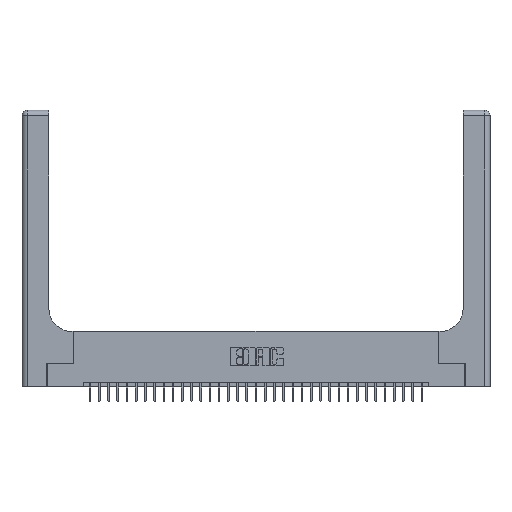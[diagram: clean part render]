
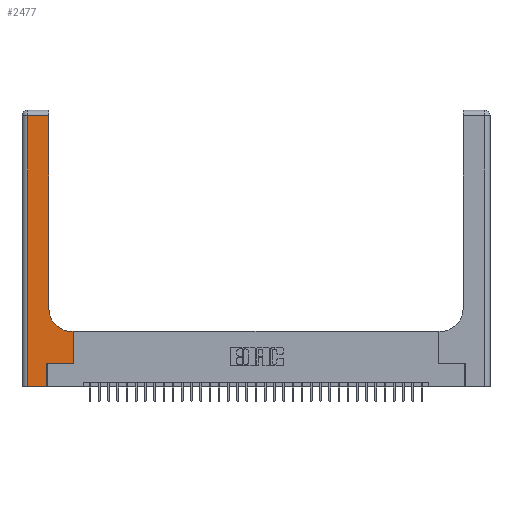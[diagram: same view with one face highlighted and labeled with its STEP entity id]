
A CAD part, top view. The second image highlights one B-rep face of the part: STEP entity #2477.
In plain terms, the highlighted planar face has unit normal (0, 0, 1).
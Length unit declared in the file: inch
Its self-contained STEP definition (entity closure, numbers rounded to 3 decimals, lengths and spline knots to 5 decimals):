
#260 = VERTEX_POINT ( 'NONE', #7170 ) ;
#374 = FACE_OUTER_BOUND ( 'NONE', #23663, .T. ) ;
#386 = VECTOR ( 'NONE', #18482, 39.37008 ) ;
#395 = ORIENTED_EDGE ( 'NONE', *, *, #7590, .T. ) ;
#452 = EDGE_CURVE ( 'NONE', #22883, #260, #27419, .T. ) ;
#1075 = DIRECTION ( 'NONE',  ( -1., 0., 0. ) ) ;
#1401 = CARTESIAN_POINT ( 'NONE',  ( 0.2915, 0.85, 0.37 ) ) ;
#1959 = EDGE_CURVE ( 'NONE', #24616, #23981, #8615, .T. ) ;
#2477 = ADVANCED_FACE ( 'NONE', ( #374 ), #9264, .F. ) ;
#3074 = EDGE_CURVE ( 'NONE', #260, #7965, #32493, .T. ) ;
#3697 = LINE ( 'NONE', #11061, #11027 ) ;
#3730 = DIRECTION ( 'NONE',  ( 0., 1., 0. ) ) ;
#3807 = CARTESIAN_POINT ( 'NONE',  ( 0.269, 0., 0.37 ) ) ;
#4621 = VECTOR ( 'NONE', #12087, 39.37008 ) ;
#4744 = EDGE_CURVE ( 'NONE', #23981, #9848, #3697, .T. ) ;
#5275 = CARTESIAN_POINT ( 'NONE',  ( 0.5585, 0.6, 0.37 ) ) ;
#6209 = CARTESIAN_POINT ( 'NONE',  ( 0.269, 0., 0.37 ) ) ;
#6589 = CARTESIAN_POINT ( 'NONE',  ( 0.5585, 0.25, 0.37 ) ) ;
#7170 = CARTESIAN_POINT ( 'NONE',  ( 0.269, 0.25, 0.37 ) ) ;
#7571 = VECTOR ( 'NONE', #3730, 39.37008 ) ;
#7590 = EDGE_CURVE ( 'NONE', #7965, #31817, #7720, .T. ) ;
#7720 = LINE ( 'NONE', #13076, #386 ) ;
#7965 = VERTEX_POINT ( 'NONE', #6589 ) ;
#8246 = VERTEX_POINT ( 'NONE', #18672 ) ;
#8615 = LINE ( 'NONE', #9902, #15818 ) ;
#9264 = PLANE ( 'NONE',  #27743 ) ;
#9478 = ORIENTED_EDGE ( 'NONE', *, *, #10785, .T. ) ;
#9848 = VERTEX_POINT ( 'NONE', #10630 ) ;
#9902 = CARTESIAN_POINT ( 'NONE',  ( 0.2915, 3., 0.37 ) ) ;
#10630 = CARTESIAN_POINT ( 'NONE',  ( 0.06, 2.94, 0.37 ) ) ;
#10785 = EDGE_CURVE ( 'NONE', #31817, #8246, #34468, .T. ) ;
#11027 = VECTOR ( 'NONE', #24602, 39.37008 ) ;
#11061 = CARTESIAN_POINT ( 'NONE',  ( 0., 2.94, 0.37 ) ) ;
#11767 = CARTESIAN_POINT ( 'NONE',  ( 0.2915, 0.6, 0.37 ) ) ;
#12087 = DIRECTION ( 'NONE',  ( 1., 0., 0. ) ) ;
#12442 = ORIENTED_EDGE ( 'NONE', *, *, #22606, .T. ) ;
#13076 = CARTESIAN_POINT ( 'NONE',  ( 0.5585, 0.25, 0.37 ) ) ;
#13103 = VECTOR ( 'NONE', #33202, 39.37008 ) ;
#14106 = ORIENTED_EDGE ( 'NONE', *, *, #3074, .T. ) ;
#14755 = CARTESIAN_POINT ( 'NONE',  ( 0.5415, 0.85, 0.37 ) ) ;
#15722 = CARTESIAN_POINT ( 'NONE',  ( 0.06, 3., 0.37 ) ) ;
#15818 = VECTOR ( 'NONE', #23325, 39.37008 ) ;
#15866 = CARTESIAN_POINT ( 'NONE',  ( 0., 0., 0.37 ) ) ;
#16409 = EDGE_CURVE ( 'NONE', #9848, #34923, #20168, .T. ) ;
#16666 = ORIENTED_EDGE ( 'NONE', *, *, #32742, .T. ) ;
#17057 = ORIENTED_EDGE ( 'NONE', *, *, #1959, .T. ) ;
#17414 = DIRECTION ( 'NONE',  ( 0., 0., -1. ) ) ;
#17468 = DIRECTION ( 'NONE',  ( 1., 0., 0. ) ) ;
#18482 = DIRECTION ( 'NONE',  ( 0., 1., 0. ) ) ;
#18672 = CARTESIAN_POINT ( 'NONE',  ( 0.5415, 0.6, 0.37 ) ) ;
#19329 = VECTOR ( 'NONE', #23834, 39.37008 ) ;
#20168 = LINE ( 'NONE', #15722, #19329 ) ;
#20722 = CIRCLE ( 'NONE', #21665, 0.25 ) ;
#21182 = CARTESIAN_POINT ( 'NONE',  ( 0.06, 0., 0.37 ) ) ;
#21290 = DIRECTION ( 'NONE',  ( 1., 0., 0. ) ) ;
#21309 = VECTOR ( 'NONE', #21290, 39.37008 ) ;
#21665 = AXIS2_PLACEMENT_3D ( 'NONE', #14755, #33498, #17468 ) ;
#22606 = EDGE_CURVE ( 'NONE', #34923, #22883, #28433, .T. ) ;
#22883 = VERTEX_POINT ( 'NONE', #6209 ) ;
#23325 = DIRECTION ( 'NONE',  ( 0., 1., 0. ) ) ;
#23663 = EDGE_LOOP ( 'NONE', ( #17057, #31309, #32971, #12442, #27571, #14106, #395, #9478, #16666 ) ) ;
#23834 = DIRECTION ( 'NONE',  ( 0., -1., 0. ) ) ;
#23981 = VERTEX_POINT ( 'NONE', #24373 ) ;
#24373 = CARTESIAN_POINT ( 'NONE',  ( 0.2915, 2.94, 0.37 ) ) ;
#24602 = DIRECTION ( 'NONE',  ( -1., 0., 0. ) ) ;
#24616 = VERTEX_POINT ( 'NONE', #1401 ) ;
#27419 = LINE ( 'NONE', #3807, #7571 ) ;
#27571 = ORIENTED_EDGE ( 'NONE', *, *, #452, .T. ) ;
#27743 = AXIS2_PLACEMENT_3D ( 'NONE', #33442, #17414, #1075 ) ;
#28190 = CARTESIAN_POINT ( 'NONE',  ( 0.269, 0.25, 0.37 ) ) ;
#28433 = LINE ( 'NONE', #15866, #21309 ) ;
#31309 = ORIENTED_EDGE ( 'NONE', *, *, #4744, .T. ) ;
#31817 = VERTEX_POINT ( 'NONE', #5275 ) ;
#32493 = LINE ( 'NONE', #28190, #4621 ) ;
#32742 = EDGE_CURVE ( 'NONE', #8246, #24616, #20722, .T. ) ;
#32971 = ORIENTED_EDGE ( 'NONE', *, *, #16409, .T. ) ;
#33202 = DIRECTION ( 'NONE',  ( -1., 0., 0. ) ) ;
#33442 = CARTESIAN_POINT ( 'NONE',  ( 0., 3., 0.37 ) ) ;
#33498 = DIRECTION ( 'NONE',  ( 0., 0., -1. ) ) ;
#34468 = LINE ( 'NONE', #11767, #13103 ) ;
#34923 = VERTEX_POINT ( 'NONE', #21182 ) ;
